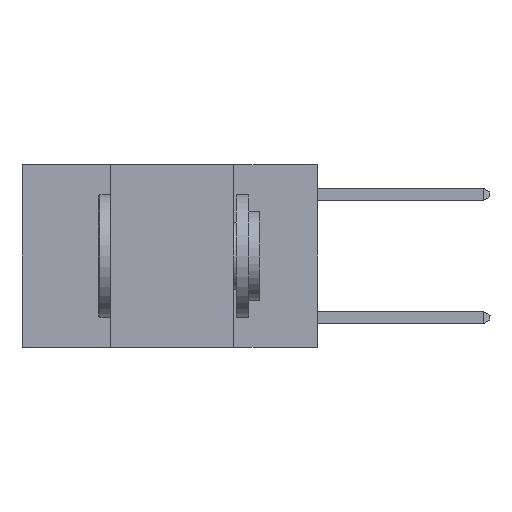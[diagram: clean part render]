
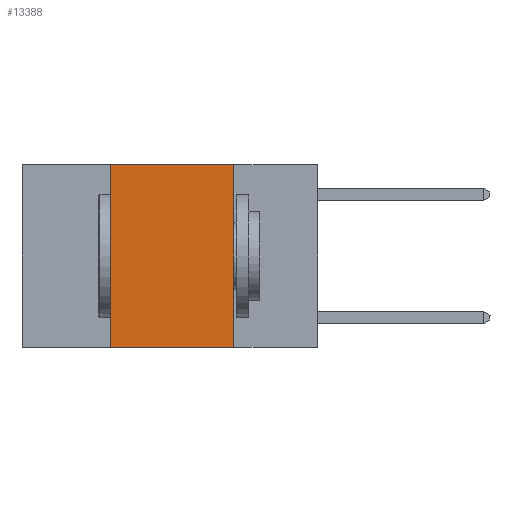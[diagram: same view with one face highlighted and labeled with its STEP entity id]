
A CAD part, left-side view. The second image highlights one B-rep face of the part: STEP entity #13388.
In plain terms, the highlighted planar face has unit normal (-1, 0, 0).
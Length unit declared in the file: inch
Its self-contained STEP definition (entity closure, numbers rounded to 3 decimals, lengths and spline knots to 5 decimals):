
#481 = VECTOR ( 'NONE', #8266, 39.37008 ) ;
#874 = DIRECTION ( 'NONE',  ( 0., 0., -1. ) ) ;
#977 = VECTOR ( 'NONE', #5291, 39.37008 ) ;
#1051 = VERTEX_POINT ( 'NONE', #12307 ) ;
#1052 = ORIENTED_EDGE ( 'NONE', *, *, #13973, .F. ) ;
#3494 = CARTESIAN_POINT ( 'NONE',  ( 0., 0.6, 0. ) ) ;
#3810 = CARTESIAN_POINT ( 'NONE',  ( 0., 0.17, 0. ) ) ;
#4077 = FACE_OUTER_BOUND ( 'NONE', #5998, .T. ) ;
#5291 = DIRECTION ( 'NONE',  ( 0., 0., -1. ) ) ;
#5941 = VECTOR ( 'NONE', #7372, 39.37008 ) ;
#5998 = EDGE_LOOP ( 'NONE', ( #13701, #1052, #7043, #12988 ) ) ;
#6040 = LINE ( 'NONE', #3494, #13208 ) ;
#6736 = EDGE_CURVE ( 'NONE', #8891, #8582, #7752, .T. ) ;
#7043 = ORIENTED_EDGE ( 'NONE', *, *, #6736, .F. ) ;
#7372 = DIRECTION ( 'NONE',  ( 0., -1., 0. ) ) ;
#7476 = EDGE_CURVE ( 'NONE', #8891, #1051, #13965, .T. ) ;
#7752 = LINE ( 'NONE', #16642, #481 ) ;
#8041 = PLANE ( 'NONE',  #10541 ) ;
#8266 = DIRECTION ( 'NONE',  ( 0., 0., 1. ) ) ;
#8329 = VERTEX_POINT ( 'NONE', #3810 ) ;
#8566 = CARTESIAN_POINT ( 'NONE',  ( 0., 0.42, 0. ) ) ;
#8582 = VERTEX_POINT ( 'NONE', #8566 ) ;
#8664 = LINE ( 'NONE', #13832, #977 ) ;
#8891 = VERTEX_POINT ( 'NONE', #9106 ) ;
#9106 = CARTESIAN_POINT ( 'NONE',  ( 0., 0.42, -0.37 ) ) ;
#9524 = DIRECTION ( 'NONE',  ( 1., 0., 0. ) ) ;
#10541 = AXIS2_PLACEMENT_3D ( 'NONE', #16472, #9524, #874 ) ;
#11599 = CARTESIAN_POINT ( 'NONE',  ( 0., 0.6, -0.37 ) ) ;
#12307 = CARTESIAN_POINT ( 'NONE',  ( 0., 0.17, -0.37 ) ) ;
#12988 = ORIENTED_EDGE ( 'NONE', *, *, #7476, .T. ) ;
#13208 = VECTOR ( 'NONE', #14852, 39.37008 ) ;
#13388 = ADVANCED_FACE ( 'NONE', ( #4077 ), #8041, .F. ) ;
#13701 = ORIENTED_EDGE ( 'NONE', *, *, #17303, .F. ) ;
#13832 = CARTESIAN_POINT ( 'NONE',  ( 0., 0.17, 0. ) ) ;
#13965 = LINE ( 'NONE', #11599, #5941 ) ;
#13973 = EDGE_CURVE ( 'NONE', #8582, #8329, #6040, .T. ) ;
#14852 = DIRECTION ( 'NONE',  ( 0., -1., 0. ) ) ;
#16472 = CARTESIAN_POINT ( 'NONE',  ( 0., 0.6, 0. ) ) ;
#16642 = CARTESIAN_POINT ( 'NONE',  ( 0., 0.42, 0. ) ) ;
#17303 = EDGE_CURVE ( 'NONE', #8329, #1051, #8664, .T. ) ;
